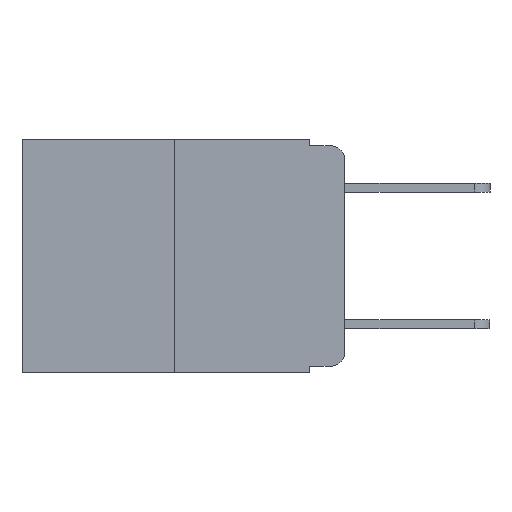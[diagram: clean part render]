
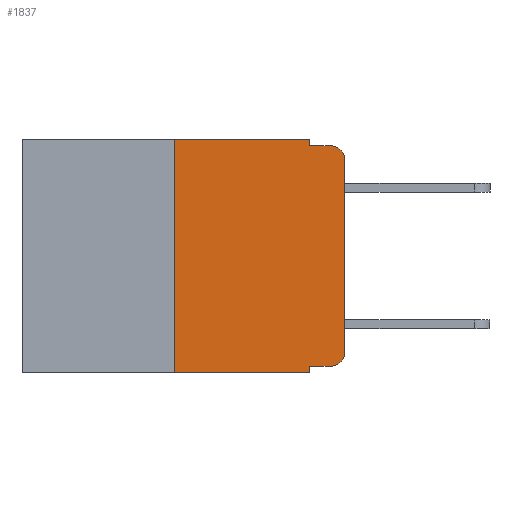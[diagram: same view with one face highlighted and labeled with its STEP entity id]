
A CAD part, left-side view. The second image highlights one B-rep face of the part: STEP entity #1837.
In plain terms, the highlighted planar face has unit normal (-1, 0, 0).
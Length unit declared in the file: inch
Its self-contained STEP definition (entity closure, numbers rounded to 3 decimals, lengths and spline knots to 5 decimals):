
#16 = LINE ( 'NONE', #1679, #5888 ) ;
#36 = VECTOR ( 'NONE', #2979, 39.37008 ) ;
#170 = EDGE_CURVE ( 'NONE', #1620, #10441, #16, .T. ) ;
#354 = CARTESIAN_POINT ( 'NONE',  ( 0., 0.473, 0. ) ) ;
#549 = ORIENTED_EDGE ( 'NONE', *, *, #2490, .T. ) ;
#674 = EDGE_CURVE ( 'NONE', #4189, #8435, #1186, .T. ) ;
#734 = VERTEX_POINT ( 'NONE', #7066 ) ;
#1186 = LINE ( 'NONE', #12805, #11832 ) ;
#1576 = CARTESIAN_POINT ( 'NONE',  ( 0., 0.051, 0. ) ) ;
#1620 = VERTEX_POINT ( 'NONE', #2048 ) ;
#1679 = CARTESIAN_POINT ( 'NONE',  ( 0., 0., 0. ) ) ;
#1837 = ADVANCED_FACE ( 'NONE', ( #3955 ), #8283, .F. ) ;
#1891 = CARTESIAN_POINT ( 'NONE',  ( 0., 0.051, 0. ) ) ;
#2048 = CARTESIAN_POINT ( 'NONE',  ( 0., 0., -0.313 ) ) ;
#2286 = EDGE_CURVE ( 'NONE', #9629, #8909, #3030, .T. ) ;
#2302 = EDGE_CURVE ( 'NONE', #4189, #5684, #10743, .T. ) ;
#2343 = EDGE_CURVE ( 'NONE', #6217, #8435, #5006, .T. ) ;
#2399 = EDGE_CURVE ( 'NONE', #734, #1620, #11864, .T. ) ;
#2453 = EDGE_CURVE ( 'NONE', #8909, #6106, #6604, .T. ) ;
#2490 = EDGE_CURVE ( 'NONE', #6217, #734, #6268, .T. ) ;
#2586 = DIRECTION ( 'NONE',  ( 0., 0., -1. ) ) ;
#2933 = ORIENTED_EDGE ( 'NONE', *, *, #2286, .F. ) ;
#2979 = DIRECTION ( 'NONE',  ( 0., -1., 0. ) ) ;
#3030 = LINE ( 'NONE', #8104, #7118 ) ;
#3507 = VECTOR ( 'NONE', #8423, 39.37008 ) ;
#3749 = DIRECTION ( 'NONE',  ( 0., 0., -1. ) ) ;
#3877 = DIRECTION ( 'NONE',  ( 1., 0., 0. ) ) ;
#3955 = FACE_OUTER_BOUND ( 'NONE', #8320, .T. ) ;
#4107 = ORIENTED_EDGE ( 'NONE', *, *, #2343, .F. ) ;
#4189 = VERTEX_POINT ( 'NONE', #6411 ) ;
#4617 = VECTOR ( 'NONE', #3749, 39.37008 ) ;
#4671 = CARTESIAN_POINT ( 'NONE',  ( 0., 0.25, 0. ) ) ;
#4872 = CARTESIAN_POINT ( 'NONE',  ( 0., 0.25, 0. ) ) ;
#5006 = LINE ( 'NONE', #1576, #4617 ) ;
#5286 = VECTOR ( 'NONE', #8206, 39.37008 ) ;
#5684 = VERTEX_POINT ( 'NONE', #4671 ) ;
#5738 = CARTESIAN_POINT ( 'NONE',  ( 0., 0.051, -0.343 ) ) ;
#5888 = VECTOR ( 'NONE', #7965, 39.37008 ) ;
#6039 = DIRECTION ( 'NONE',  ( -1., 0., 0. ) ) ;
#6106 = VERTEX_POINT ( 'NONE', #12086 ) ;
#6217 = VERTEX_POINT ( 'NONE', #9838 ) ;
#6246 = EDGE_CURVE ( 'NONE', #10441, #6106, #6976, .T. ) ;
#6268 = LINE ( 'NONE', #12558, #36 ) ;
#6291 = DIRECTION ( 'NONE',  ( -1., 0., 0. ) ) ;
#6411 = CARTESIAN_POINT ( 'NONE',  ( 0., 0.25, -0.343 ) ) ;
#6604 = LINE ( 'NONE', #12518, #3507 ) ;
#6675 = ORIENTED_EDGE ( 'NONE', *, *, #7341, .F. ) ;
#6760 = CARTESIAN_POINT ( 'NONE',  ( 0., 0., -0.03 ) ) ;
#6976 = CIRCLE ( 'NONE', #10284, 0.02 ) ;
#7066 = CARTESIAN_POINT ( 'NONE',  ( 0., 0.02, -0.333 ) ) ;
#7118 = VECTOR ( 'NONE', #2586, 39.37008 ) ;
#7290 = CARTESIAN_POINT ( 'NONE',  ( 0., 0.473, 0. ) ) ;
#7315 = ORIENTED_EDGE ( 'NONE', *, *, #170, .T. ) ;
#7341 = EDGE_CURVE ( 'NONE', #5684, #9629, #8416, .T. ) ;
#7965 = DIRECTION ( 'NONE',  ( 0., 0., 1. ) ) ;
#8104 = CARTESIAN_POINT ( 'NONE',  ( 0., 0.051, 0. ) ) ;
#8174 = CARTESIAN_POINT ( 'NONE',  ( 0., 0.051, -0.01 ) ) ;
#8206 = DIRECTION ( 'NONE',  ( 0., -1., 0. ) ) ;
#8248 = ORIENTED_EDGE ( 'NONE', *, *, #6246, .T. ) ;
#8283 = PLANE ( 'NONE',  #11694 ) ;
#8320 = EDGE_LOOP ( 'NONE', ( #7315, #8248, #12271, #2933, #6675, #12155, #11050, #4107, #549, #11666 ) ) ;
#8416 = LINE ( 'NONE', #354, #5286 ) ;
#8423 = DIRECTION ( 'NONE',  ( 0., -1., 0. ) ) ;
#8435 = VERTEX_POINT ( 'NONE', #5738 ) ;
#8909 = VERTEX_POINT ( 'NONE', #8174 ) ;
#9019 = DIRECTION ( 'NONE',  ( 0., 0., 1. ) ) ;
#9629 = VERTEX_POINT ( 'NONE', #1891 ) ;
#9838 = CARTESIAN_POINT ( 'NONE',  ( 0., 0.051, -0.333 ) ) ;
#10284 = AXIS2_PLACEMENT_3D ( 'NONE', #11479, #6039, #12277 ) ;
#10441 = VERTEX_POINT ( 'NONE', #6760 ) ;
#10502 = VECTOR ( 'NONE', #9019, 39.37008 ) ;
#10743 = LINE ( 'NONE', #4872, #10502 ) ;
#10852 = DIRECTION ( 'NONE',  ( 0., 0., -1. ) ) ;
#11050 = ORIENTED_EDGE ( 'NONE', *, *, #674, .T. ) ;
#11479 = CARTESIAN_POINT ( 'NONE',  ( 0., 0.02, -0.03 ) ) ;
#11499 = DIRECTION ( 'NONE',  ( 0., -1., 0. ) ) ;
#11655 = CARTESIAN_POINT ( 'NONE',  ( 0., 0.02, -0.313 ) ) ;
#11666 = ORIENTED_EDGE ( 'NONE', *, *, #2399, .T. ) ;
#11694 = AXIS2_PLACEMENT_3D ( 'NONE', #7290, #3877, #10852 ) ;
#11832 = VECTOR ( 'NONE', #11499, 39.37008 ) ;
#11837 = AXIS2_PLACEMENT_3D ( 'NONE', #11655, #6291, #12454 ) ;
#11864 = CIRCLE ( 'NONE', #11837, 0.02 ) ;
#12086 = CARTESIAN_POINT ( 'NONE',  ( 0., 0.02, -0.01 ) ) ;
#12155 = ORIENTED_EDGE ( 'NONE', *, *, #2302, .F. ) ;
#12271 = ORIENTED_EDGE ( 'NONE', *, *, #2453, .F. ) ;
#12277 = DIRECTION ( 'NONE',  ( 0., 0., -1. ) ) ;
#12454 = DIRECTION ( 'NONE',  ( 0., 0., -1. ) ) ;
#12518 = CARTESIAN_POINT ( 'NONE',  ( 0., 0.051, -0.01 ) ) ;
#12558 = CARTESIAN_POINT ( 'NONE',  ( 0., 0.051, -0.333 ) ) ;
#12805 = CARTESIAN_POINT ( 'NONE',  ( 0., 0.473, -0.343 ) ) ;
